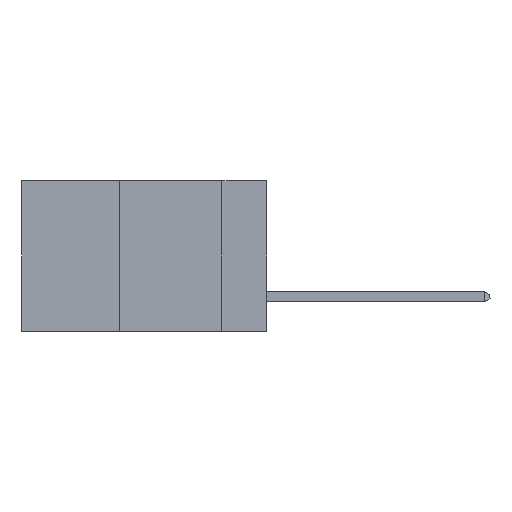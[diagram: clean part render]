
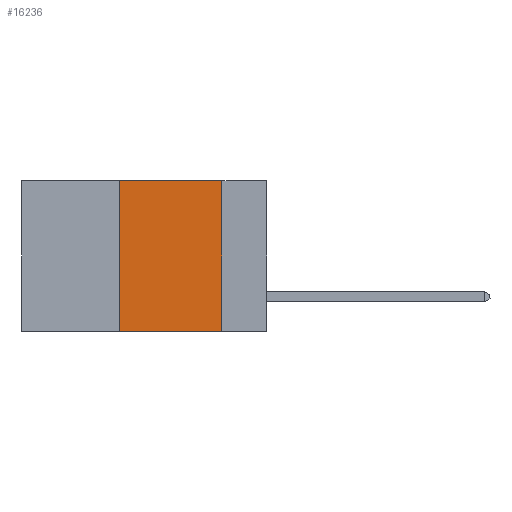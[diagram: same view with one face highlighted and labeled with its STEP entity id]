
A CAD part, left-side view. The second image highlights one B-rep face of the part: STEP entity #16236.
In plain terms, the highlighted planar face has unit normal (-1, 0, 0).
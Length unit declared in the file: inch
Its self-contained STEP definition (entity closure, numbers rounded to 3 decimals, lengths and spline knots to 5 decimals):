
#380 = CARTESIAN_POINT ( 'NONE',  ( 0., 0.11, 0. ) ) ;
#656 = CARTESIAN_POINT ( 'NONE',  ( 0., 0.11, -0.37 ) ) ;
#969 = DIRECTION ( 'NONE',  ( 0., -1., 0. ) ) ;
#1359 = CARTESIAN_POINT ( 'NONE',  ( 0., 0.11, 0. ) ) ;
#1908 = EDGE_CURVE ( 'NONE', #5231, #13311, #23136, .T. ) ;
#2637 = DIRECTION ( 'NONE',  ( 0., 0., -1. ) ) ;
#4235 = CARTESIAN_POINT ( 'NONE',  ( 0., 0.6, -0.37 ) ) ;
#4749 = VERTEX_POINT ( 'NONE', #26611 ) ;
#5181 = ORIENTED_EDGE ( 'NONE', *, *, #34512, .F. ) ;
#5231 = VERTEX_POINT ( 'NONE', #26298 ) ;
#6316 = VECTOR ( 'NONE', #969, 39.37008 ) ;
#8027 = DIRECTION ( 'NONE',  ( 0., 0., -1. ) ) ;
#8413 = LINE ( 'NONE', #4235, #6316 ) ;
#11341 = LINE ( 'NONE', #1359, #13361 ) ;
#13311 = VERTEX_POINT ( 'NONE', #380 ) ;
#13361 = VECTOR ( 'NONE', #8027, 39.37008 ) ;
#13374 = VECTOR ( 'NONE', #42183, 39.37008 ) ;
#15338 = VERTEX_POINT ( 'NONE', #656 ) ;
#16236 = ADVANCED_FACE ( 'NONE', ( #39422 ), #38373, .F. ) ;
#16872 = EDGE_LOOP ( 'NONE', ( #20627, #35709, #5181, #33171 ) ) ;
#19164 = CARTESIAN_POINT ( 'NONE',  ( 0., 0.6, 0. ) ) ;
#20627 = ORIENTED_EDGE ( 'NONE', *, *, #31053, .F. ) ;
#22429 = DIRECTION ( 'NONE',  ( 1., 0., 0. ) ) ;
#22810 = VECTOR ( 'NONE', #26230, 39.37008 ) ;
#23136 = LINE ( 'NONE', #26243, #13374 ) ;
#23835 = LINE ( 'NONE', #38940, #22810 ) ;
#26230 = DIRECTION ( 'NONE',  ( 0., 0., 1. ) ) ;
#26243 = CARTESIAN_POINT ( 'NONE',  ( 0., 0.6, 0. ) ) ;
#26298 = CARTESIAN_POINT ( 'NONE',  ( 0., 0.36, 0. ) ) ;
#26611 = CARTESIAN_POINT ( 'NONE',  ( 0., 0.36, -0.37 ) ) ;
#31053 = EDGE_CURVE ( 'NONE', #13311, #15338, #11341, .T. ) ;
#33171 = ORIENTED_EDGE ( 'NONE', *, *, #35298, .T. ) ;
#33700 = AXIS2_PLACEMENT_3D ( 'NONE', #19164, #22429, #2637 ) ;
#34512 = EDGE_CURVE ( 'NONE', #4749, #5231, #23835, .T. ) ;
#35298 = EDGE_CURVE ( 'NONE', #4749, #15338, #8413, .T. ) ;
#35709 = ORIENTED_EDGE ( 'NONE', *, *, #1908, .F. ) ;
#38373 = PLANE ( 'NONE',  #33700 ) ;
#38940 = CARTESIAN_POINT ( 'NONE',  ( 0., 0.36, 0. ) ) ;
#39422 = FACE_OUTER_BOUND ( 'NONE', #16872, .T. ) ;
#42183 = DIRECTION ( 'NONE',  ( 0., -1., 0. ) ) ;
